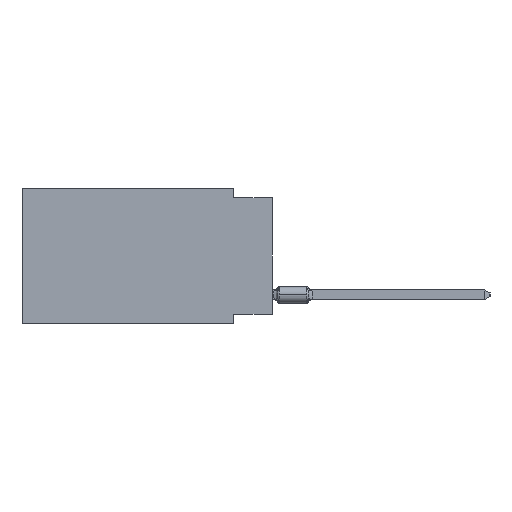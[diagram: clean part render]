
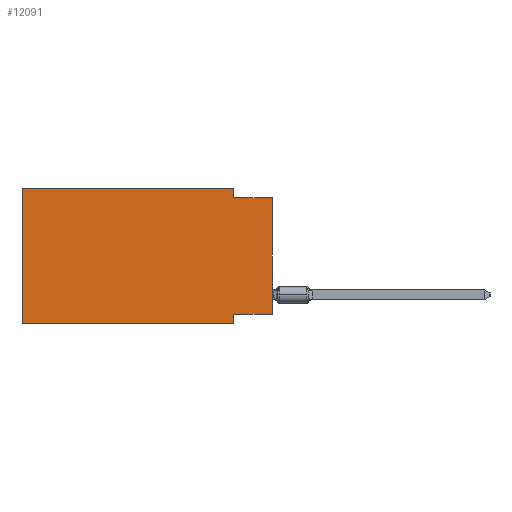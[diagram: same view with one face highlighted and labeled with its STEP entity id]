
A CAD part, left-side view. The second image highlights one B-rep face of the part: STEP entity #12091.
In plain terms, the highlighted planar face has unit normal (-1, 0, 0).
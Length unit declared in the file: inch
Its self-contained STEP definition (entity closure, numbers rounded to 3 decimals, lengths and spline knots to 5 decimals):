
#24 = VERTEX_POINT ( 'NONE', #33577 ) ;
#45 = ORIENTED_EDGE ( 'NONE', *, *, #20480, .F. ) ;
#1183 = DIRECTION ( 'NONE',  ( 0., 0., -1. ) ) ;
#1361 = LINE ( 'NONE', #11694, #30824 ) ;
#1986 = VERTEX_POINT ( 'NONE', #29116 ) ;
#2300 = VECTOR ( 'NONE', #28950, 39.37008 ) ;
#2782 = VERTEX_POINT ( 'NONE', #25770 ) ;
#2906 = DIRECTION ( 'NONE',  ( 0., 0., -1. ) ) ;
#2921 = VECTOR ( 'NONE', #6837, 39.37008 ) ;
#3813 = EDGE_CURVE ( 'NONE', #29967, #23985, #1361, .T. ) ;
#4101 = ORIENTED_EDGE ( 'NONE', *, *, #19458, .F. ) ;
#4252 = DIRECTION ( 'NONE',  ( 0., 1., 0. ) ) ;
#4323 = VERTEX_POINT ( 'NONE', #31139 ) ;
#5618 = CARTESIAN_POINT ( 'NONE',  ( 0., 0.1, -0.35 ) ) ;
#6192 = CARTESIAN_POINT ( 'NONE',  ( 0., 0.1, 0. ) ) ;
#6472 = CARTESIAN_POINT ( 'NONE',  ( 0., 0., -0.325 ) ) ;
#6837 = DIRECTION ( 'NONE',  ( 0., 0., 1. ) ) ;
#8270 = EDGE_CURVE ( 'NONE', #24, #23985, #21062, .T. ) ;
#8536 = CARTESIAN_POINT ( 'NONE',  ( 0., 0., 0. ) ) ;
#8558 = LINE ( 'NONE', #6192, #10696 ) ;
#8735 = DIRECTION ( 'NONE',  ( 0., 0., -1. ) ) ;
#9221 = CARTESIAN_POINT ( 'NONE',  ( 0., 0.645, 0. ) ) ;
#9615 = EDGE_LOOP ( 'NONE', ( #32885, #4101, #45, #14738, #32336, #25298, #16310, #10497 ) ) ;
#10497 = ORIENTED_EDGE ( 'NONE', *, *, #11690, .F. ) ;
#10696 = VECTOR ( 'NONE', #8735, 39.37008 ) ;
#11426 = LINE ( 'NONE', #9221, #2921 ) ;
#11690 = EDGE_CURVE ( 'NONE', #11723, #24, #32634, .T. ) ;
#11694 = CARTESIAN_POINT ( 'NONE',  ( 0., 0.645, -0.35 ) ) ;
#11723 = VERTEX_POINT ( 'NONE', #27208 ) ;
#12091 = ADVANCED_FACE ( 'NONE', ( #27493 ), #22391, .F. ) ;
#12700 = EDGE_CURVE ( 'NONE', #29967, #4323, #11426, .T. ) ;
#12848 = CARTESIAN_POINT ( 'NONE',  ( 0., 0.1, -0.35 ) ) ;
#14415 = DIRECTION ( 'NONE',  ( 0., -1., 0. ) ) ;
#14738 = ORIENTED_EDGE ( 'NONE', *, *, #25809, .F. ) ;
#16173 = CARTESIAN_POINT ( 'NONE',  ( 0., 0.645, -0.35 ) ) ;
#16211 = DIRECTION ( 'NONE',  ( 0., -1., 0. ) ) ;
#16310 = ORIENTED_EDGE ( 'NONE', *, *, #8270, .F. ) ;
#16540 = LINE ( 'NONE', #26545, #31593 ) ;
#16784 = CARTESIAN_POINT ( 'NONE',  ( 0., 0.645, 0. ) ) ;
#19458 = EDGE_CURVE ( 'NONE', #2782, #25686, #33400, .T. ) ;
#20480 = EDGE_CURVE ( 'NONE', #1986, #2782, #8558, .T. ) ;
#21062 = LINE ( 'NONE', #5618, #30748 ) ;
#21531 = VECTOR ( 'NONE', #16211, 39.37008 ) ;
#22391 = PLANE ( 'NONE',  #27299 ) ;
#22542 = DIRECTION ( 'NONE',  ( 1., 0., 0. ) ) ;
#23858 = CARTESIAN_POINT ( 'NONE',  ( 0., 0., -0.025 ) ) ;
#23985 = VERTEX_POINT ( 'NONE', #12848 ) ;
#25298 = ORIENTED_EDGE ( 'NONE', *, *, #3813, .T. ) ;
#25686 = VERTEX_POINT ( 'NONE', #23858 ) ;
#25770 = CARTESIAN_POINT ( 'NONE',  ( 0., 0.1, -0.025 ) ) ;
#25809 = EDGE_CURVE ( 'NONE', #4323, #1986, #16540, .T. ) ;
#25857 = EDGE_CURVE ( 'NONE', #11723, #25686, #26050, .T. ) ;
#26050 = LINE ( 'NONE', #8536, #2300 ) ;
#26545 = CARTESIAN_POINT ( 'NONE',  ( 0., 0.645, 0. ) ) ;
#27208 = CARTESIAN_POINT ( 'NONE',  ( 0., 0., -0.325 ) ) ;
#27299 = AXIS2_PLACEMENT_3D ( 'NONE', #16784, #22542, #1183 ) ;
#27493 = FACE_OUTER_BOUND ( 'NONE', #9615, .T. ) ;
#28950 = DIRECTION ( 'NONE',  ( 0., 0., 1. ) ) ;
#29116 = CARTESIAN_POINT ( 'NONE',  ( 0., 0.1, 0. ) ) ;
#29451 = VECTOR ( 'NONE', #4252, 39.37008 ) ;
#29967 = VERTEX_POINT ( 'NONE', #16173 ) ;
#30679 = CARTESIAN_POINT ( 'NONE',  ( 0., 0., -0.025 ) ) ;
#30748 = VECTOR ( 'NONE', #2906, 39.37008 ) ;
#30824 = VECTOR ( 'NONE', #14415, 39.37008 ) ;
#31139 = CARTESIAN_POINT ( 'NONE',  ( 0., 0.645, 0. ) ) ;
#31157 = DIRECTION ( 'NONE',  ( 0., -1., 0. ) ) ;
#31593 = VECTOR ( 'NONE', #31157, 39.37008 ) ;
#32336 = ORIENTED_EDGE ( 'NONE', *, *, #12700, .F. ) ;
#32634 = LINE ( 'NONE', #6472, #29451 ) ;
#32885 = ORIENTED_EDGE ( 'NONE', *, *, #25857, .T. ) ;
#33400 = LINE ( 'NONE', #30679, #21531 ) ;
#33577 = CARTESIAN_POINT ( 'NONE',  ( 0., 0.1, -0.325 ) ) ;
